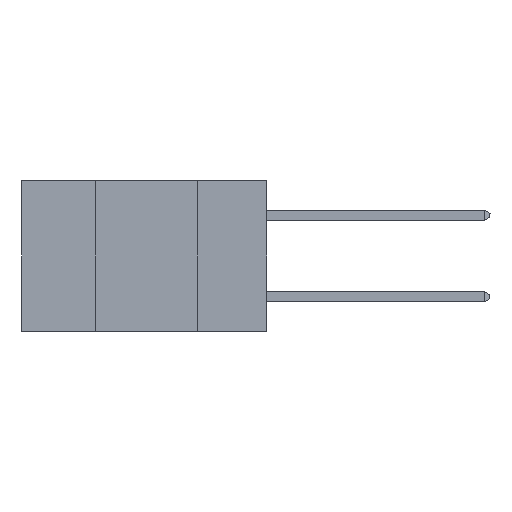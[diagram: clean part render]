
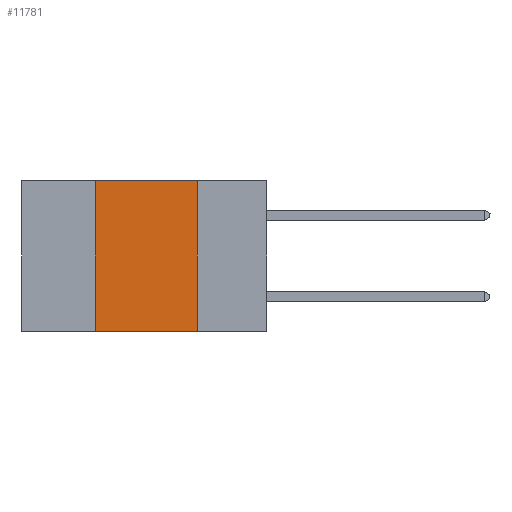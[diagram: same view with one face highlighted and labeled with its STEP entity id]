
A CAD part, left-side view. The second image highlights one B-rep face of the part: STEP entity #11781.
In plain terms, the highlighted planar face has unit normal (-1, 0, 0).
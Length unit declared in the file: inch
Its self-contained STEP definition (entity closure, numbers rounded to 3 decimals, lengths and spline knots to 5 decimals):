
#495 = ORIENTED_EDGE ( 'NONE', *, *, #11531, .T. ) ;
#1317 = CARTESIAN_POINT ( 'NONE',  ( 0., 0.6, 0. ) ) ;
#1640 = PLANE ( 'NONE',  #12831 ) ;
#1702 = CARTESIAN_POINT ( 'NONE',  ( 0., 0.17, 0. ) ) ;
#2324 = EDGE_CURVE ( 'NONE', #2828, #9622, #10852, .T. ) ;
#2624 = ORIENTED_EDGE ( 'NONE', *, *, #18288, .F. ) ;
#2828 = VERTEX_POINT ( 'NONE', #13150 ) ;
#4024 = VECTOR ( 'NONE', #12424, 39.37008 ) ;
#4223 = CARTESIAN_POINT ( 'NONE',  ( 0., 0.6, 0. ) ) ;
#5584 = ORIENTED_EDGE ( 'NONE', *, *, #15423, .F. ) ;
#6033 = CARTESIAN_POINT ( 'NONE',  ( 0., 0.17, -0.37 ) ) ;
#6382 = VECTOR ( 'NONE', #9185, 39.37008 ) ;
#7536 = VECTOR ( 'NONE', #10613, 39.37008 ) ;
#8065 = DIRECTION ( 'NONE',  ( 1., 0., 0. ) ) ;
#8969 = CARTESIAN_POINT ( 'NONE',  ( 0., 0.6, -0.37 ) ) ;
#9185 = DIRECTION ( 'NONE',  ( 0., 0., 1. ) ) ;
#9622 = VERTEX_POINT ( 'NONE', #15085 ) ;
#10324 = CARTESIAN_POINT ( 'NONE',  ( 0., 0.17, 0. ) ) ;
#10613 = DIRECTION ( 'NONE',  ( 0., -1., 0. ) ) ;
#10852 = LINE ( 'NONE', #17603, #6382 ) ;
#11054 = DIRECTION ( 'NONE',  ( 0., 0., -1. ) ) ;
#11531 = EDGE_CURVE ( 'NONE', #2828, #18176, #18805, .T. ) ;
#11606 = FACE_OUTER_BOUND ( 'NONE', #15392, .T. ) ;
#11781 = ADVANCED_FACE ( 'NONE', ( #11606 ), #1640, .F. ) ;
#12412 = VECTOR ( 'NONE', #21626, 39.37008 ) ;
#12424 = DIRECTION ( 'NONE',  ( 0., -1., 0. ) ) ;
#12831 = AXIS2_PLACEMENT_3D ( 'NONE', #1317, #8065, #11054 ) ;
#13150 = CARTESIAN_POINT ( 'NONE',  ( 0., 0.42, -0.37 ) ) ;
#14192 = LINE ( 'NONE', #4223, #4024 ) ;
#15085 = CARTESIAN_POINT ( 'NONE',  ( 0., 0.42, 0. ) ) ;
#15103 = LINE ( 'NONE', #1702, #12412 ) ;
#15392 = EDGE_LOOP ( 'NONE', ( #2624, #5584, #21600, #495 ) ) ;
#15423 = EDGE_CURVE ( 'NONE', #9622, #16564, #14192, .T. ) ;
#16564 = VERTEX_POINT ( 'NONE', #10324 ) ;
#17603 = CARTESIAN_POINT ( 'NONE',  ( 0., 0.42, 0. ) ) ;
#18176 = VERTEX_POINT ( 'NONE', #6033 ) ;
#18288 = EDGE_CURVE ( 'NONE', #16564, #18176, #15103, .T. ) ;
#18805 = LINE ( 'NONE', #8969, #7536 ) ;
#21600 = ORIENTED_EDGE ( 'NONE', *, *, #2324, .F. ) ;
#21626 = DIRECTION ( 'NONE',  ( 0., 0., -1. ) ) ;
